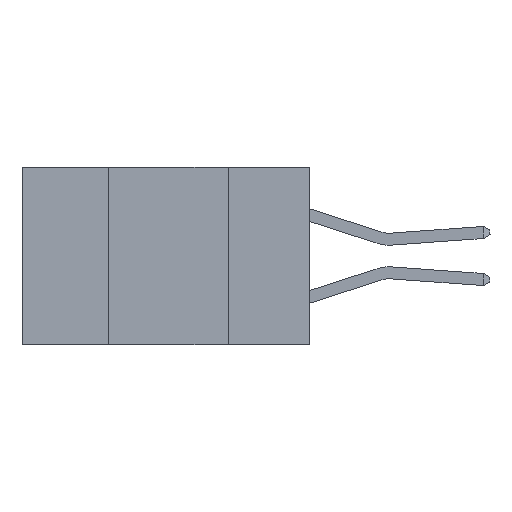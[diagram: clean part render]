
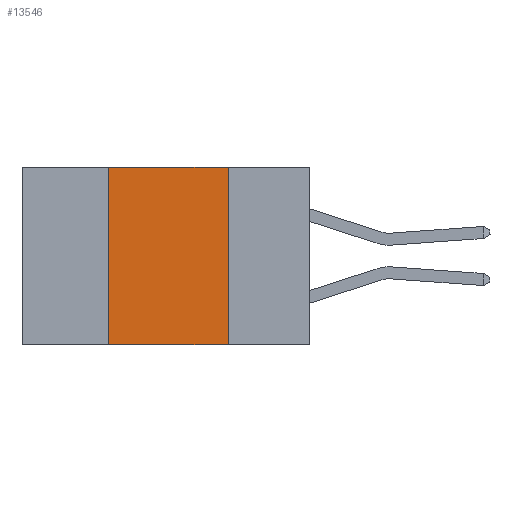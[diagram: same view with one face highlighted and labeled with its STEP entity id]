
A CAD part, left-side view. The second image highlights one B-rep face of the part: STEP entity #13546.
In plain terms, the highlighted planar face has unit normal (-1, 0, 0).
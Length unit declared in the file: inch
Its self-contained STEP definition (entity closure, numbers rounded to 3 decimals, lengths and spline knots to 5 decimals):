
#624 = CARTESIAN_POINT ( 'NONE',  ( 0., 0.6, 0. ) ) ;
#2971 = VERTEX_POINT ( 'NONE', #6678 ) ;
#4224 = CARTESIAN_POINT ( 'NONE',  ( 0., 0.42, 0. ) ) ;
#4856 = DIRECTION ( 'NONE',  ( 0., 0., -1. ) ) ;
#5355 = CARTESIAN_POINT ( 'NONE',  ( 0., 0.42, 0. ) ) ;
#6250 = EDGE_CURVE ( 'NONE', #16158, #18656, #24780, .T. ) ;
#6551 = VECTOR ( 'NONE', #10667, 39.37008 ) ;
#6678 = CARTESIAN_POINT ( 'NONE',  ( 0., 0.17, 0. ) ) ;
#8025 = CARTESIAN_POINT ( 'NONE',  ( 0., 0.6, 0. ) ) ;
#8163 = VERTEX_POINT ( 'NONE', #18437 ) ;
#8836 = CARTESIAN_POINT ( 'NONE',  ( 0., 0.42, -0.37 ) ) ;
#8863 = DIRECTION ( 'NONE',  ( 1., 0., 0. ) ) ;
#9907 = EDGE_CURVE ( 'NONE', #2971, #8163, #14884, .T. ) ;
#10667 = DIRECTION ( 'NONE',  ( 0., 0., 1. ) ) ;
#11379 = LINE ( 'NONE', #8025, #24052 ) ;
#12350 = FACE_OUTER_BOUND ( 'NONE', #21829, .T. ) ;
#13439 = PLANE ( 'NONE',  #23713 ) ;
#13546 = ADVANCED_FACE ( 'NONE', ( #12350 ), #13439, .F. ) ;
#14054 = ORIENTED_EDGE ( 'NONE', *, *, #6250, .F. ) ;
#14705 = EDGE_CURVE ( 'NONE', #16158, #8163, #19988, .T. ) ;
#14884 = LINE ( 'NONE', #22413, #16225 ) ;
#16158 = VERTEX_POINT ( 'NONE', #8836 ) ;
#16225 = VECTOR ( 'NONE', #26619, 39.37008 ) ;
#18339 = ORIENTED_EDGE ( 'NONE', *, *, #26662, .F. ) ;
#18437 = CARTESIAN_POINT ( 'NONE',  ( 0., 0.17, -0.37 ) ) ;
#18656 = VERTEX_POINT ( 'NONE', #5355 ) ;
#19988 = LINE ( 'NONE', #23312, #24525 ) ;
#20154 = DIRECTION ( 'NONE',  ( 0., -1., 0. ) ) ;
#21829 = EDGE_LOOP ( 'NONE', ( #25597, #18339, #14054, #22986 ) ) ;
#22413 = CARTESIAN_POINT ( 'NONE',  ( 0., 0.17, 0. ) ) ;
#22986 = ORIENTED_EDGE ( 'NONE', *, *, #14705, .T. ) ;
#23312 = CARTESIAN_POINT ( 'NONE',  ( 0., 0.6, -0.37 ) ) ;
#23713 = AXIS2_PLACEMENT_3D ( 'NONE', #624, #8863, #4856 ) ;
#24052 = VECTOR ( 'NONE', #20154, 39.37008 ) ;
#24525 = VECTOR ( 'NONE', #25426, 39.37008 ) ;
#24780 = LINE ( 'NONE', #4224, #6551 ) ;
#25426 = DIRECTION ( 'NONE',  ( 0., -1., 0. ) ) ;
#25597 = ORIENTED_EDGE ( 'NONE', *, *, #9907, .F. ) ;
#26619 = DIRECTION ( 'NONE',  ( 0., 0., -1. ) ) ;
#26662 = EDGE_CURVE ( 'NONE', #18656, #2971, #11379, .T. ) ;
